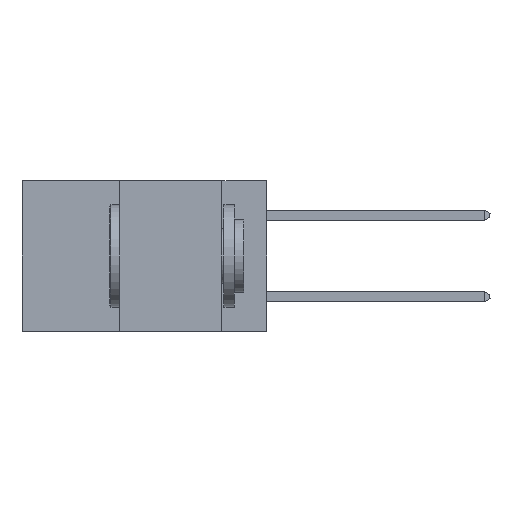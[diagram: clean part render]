
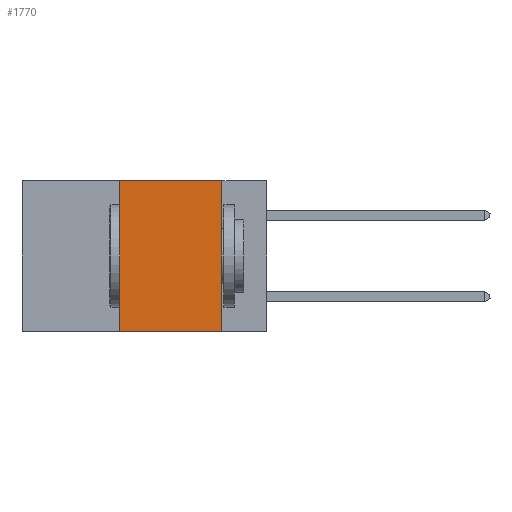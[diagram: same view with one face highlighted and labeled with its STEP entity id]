
A CAD part, left-side view. The second image highlights one B-rep face of the part: STEP entity #1770.
In plain terms, the highlighted planar face has unit normal (-1, 0, 0).
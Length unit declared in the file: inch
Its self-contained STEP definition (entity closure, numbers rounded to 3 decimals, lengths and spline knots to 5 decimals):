
#339 = CARTESIAN_POINT ( 'NONE',  ( 0., 0.11, 0. ) ) ;
#519 = LINE ( 'NONE', #6656, #2820 ) ;
#798 = EDGE_CURVE ( 'NONE', #1757, #11331, #14499, .T. ) ;
#1371 = DIRECTION ( 'NONE',  ( 0., -1., 0. ) ) ;
#1757 = VERTEX_POINT ( 'NONE', #6896 ) ;
#1770 = ADVANCED_FACE ( 'NONE', ( #14327 ), #7317, .F. ) ;
#2457 = EDGE_CURVE ( 'NONE', #9700, #14321, #15595, .T. ) ;
#2633 = AXIS2_PLACEMENT_3D ( 'NONE', #10956, #6077, #14459 ) ;
#2721 = ORIENTED_EDGE ( 'NONE', *, *, #2457, .F. ) ;
#2820 = VECTOR ( 'NONE', #1371, 39.37008 ) ;
#2949 = CARTESIAN_POINT ( 'NONE',  ( 0., 0.36, 0. ) ) ;
#3920 = CARTESIAN_POINT ( 'NONE',  ( 0., 0.11, 0. ) ) ;
#4124 = ORIENTED_EDGE ( 'NONE', *, *, #798, .F. ) ;
#4548 = EDGE_LOOP ( 'NONE', ( #2721, #10296, #4124, #14097 ) ) ;
#4782 = VECTOR ( 'NONE', #11086, 39.37008 ) ;
#6077 = DIRECTION ( 'NONE',  ( 1., 0., 0. ) ) ;
#6325 = EDGE_CURVE ( 'NONE', #1757, #14321, #6562, .T. ) ;
#6562 = LINE ( 'NONE', #12371, #9475 ) ;
#6656 = CARTESIAN_POINT ( 'NONE',  ( 0., 0.6, 0. ) ) ;
#6896 = CARTESIAN_POINT ( 'NONE',  ( 0., 0.36, -0.37 ) ) ;
#7317 = PLANE ( 'NONE',  #2633 ) ;
#8576 = CARTESIAN_POINT ( 'NONE',  ( 0., 0.36, 0. ) ) ;
#9475 = VECTOR ( 'NONE', #13544, 39.37008 ) ;
#9700 = VERTEX_POINT ( 'NONE', #339 ) ;
#10296 = ORIENTED_EDGE ( 'NONE', *, *, #11839, .F. ) ;
#10472 = DIRECTION ( 'NONE',  ( 0., 0., -1. ) ) ;
#10956 = CARTESIAN_POINT ( 'NONE',  ( 0., 0.6, 0. ) ) ;
#11058 = CARTESIAN_POINT ( 'NONE',  ( 0., 0.11, -0.37 ) ) ;
#11086 = DIRECTION ( 'NONE',  ( 0., 0., 1. ) ) ;
#11331 = VERTEX_POINT ( 'NONE', #2949 ) ;
#11839 = EDGE_CURVE ( 'NONE', #11331, #9700, #519, .T. ) ;
#12371 = CARTESIAN_POINT ( 'NONE',  ( 0., 0.6, -0.37 ) ) ;
#13544 = DIRECTION ( 'NONE',  ( 0., -1., 0. ) ) ;
#14097 = ORIENTED_EDGE ( 'NONE', *, *, #6325, .T. ) ;
#14321 = VERTEX_POINT ( 'NONE', #11058 ) ;
#14327 = FACE_OUTER_BOUND ( 'NONE', #4548, .T. ) ;
#14459 = DIRECTION ( 'NONE',  ( 0., 0., -1. ) ) ;
#14499 = LINE ( 'NONE', #8576, #4782 ) ;
#15213 = VECTOR ( 'NONE', #10472, 39.37008 ) ;
#15595 = LINE ( 'NONE', #3920, #15213 ) ;
